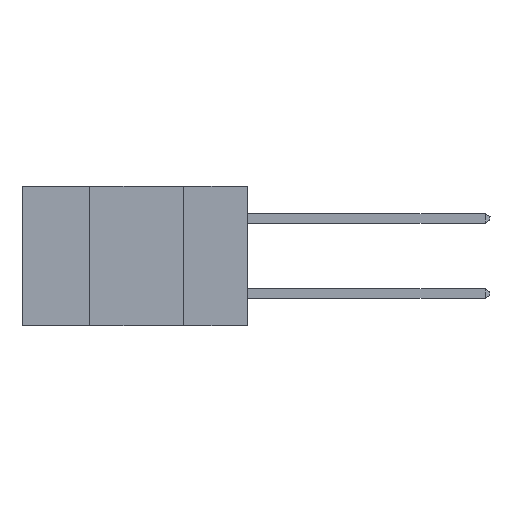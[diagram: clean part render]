
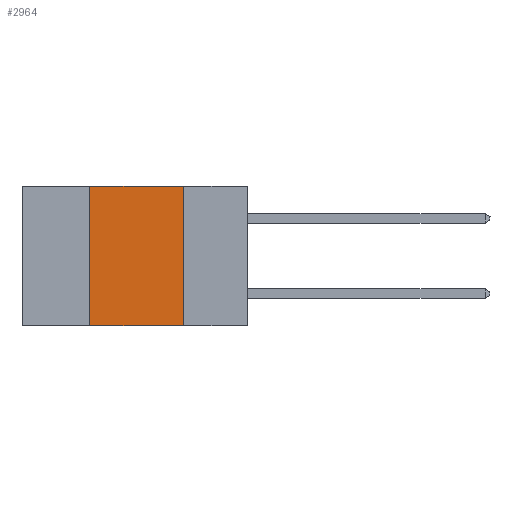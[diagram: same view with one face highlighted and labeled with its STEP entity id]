
A CAD part, left-side view. The second image highlights one B-rep face of the part: STEP entity #2964.
In plain terms, the highlighted planar face has unit normal (-1, 0, 0).
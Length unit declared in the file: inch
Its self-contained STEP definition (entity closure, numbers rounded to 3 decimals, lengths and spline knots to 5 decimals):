
#119 = DIRECTION ( 'NONE',  ( 0., -1., 0. ) ) ;
#792 = VECTOR ( 'NONE', #4960, 39.37008 ) ;
#814 = PLANE ( 'NONE',  #4036 ) ;
#1105 = ORIENTED_EDGE ( 'NONE', *, *, #10908, .F. ) ;
#1629 = EDGE_CURVE ( 'NONE', #7614, #4174, #7668, .T. ) ;
#1690 = DIRECTION ( 'NONE',  ( 0., -1., 0. ) ) ;
#1765 = DIRECTION ( 'NONE',  ( 1., 0., 0. ) ) ;
#1838 = CARTESIAN_POINT ( 'NONE',  ( 0., 0.42, 0. ) ) ;
#2436 = ORIENTED_EDGE ( 'NONE', *, *, #1629, .F. ) ;
#2517 = EDGE_CURVE ( 'NONE', #7547, #3492, #9523, .T. ) ;
#2719 = FACE_OUTER_BOUND ( 'NONE', #5638, .T. ) ;
#2964 = ADVANCED_FACE ( 'NONE', ( #2719 ), #814, .F. ) ;
#3097 = CARTESIAN_POINT ( 'NONE',  ( 0., 0.17, -0.37 ) ) ;
#3125 = CARTESIAN_POINT ( 'NONE',  ( 0., 0.42, -0.37 ) ) ;
#3251 = DIRECTION ( 'NONE',  ( 0., 0., 1. ) ) ;
#3470 = VECTOR ( 'NONE', #119, 39.37008 ) ;
#3492 = VERTEX_POINT ( 'NONE', #4029 ) ;
#3635 = EDGE_CURVE ( 'NONE', #7614, #3492, #7477, .T. ) ;
#4029 = CARTESIAN_POINT ( 'NONE',  ( 0., 0.17, -0.37 ) ) ;
#4036 = AXIS2_PLACEMENT_3D ( 'NONE', #8968, #1765, #5299 ) ;
#4174 = VERTEX_POINT ( 'NONE', #1838 ) ;
#4931 = ORIENTED_EDGE ( 'NONE', *, *, #3635, .T. ) ;
#4960 = DIRECTION ( 'NONE',  ( 0., 0., -1. ) ) ;
#5299 = DIRECTION ( 'NONE',  ( 0., 0., -1. ) ) ;
#5638 = EDGE_LOOP ( 'NONE', ( #11481, #1105, #2436, #4931 ) ) ;
#6113 = LINE ( 'NONE', #7183, #11177 ) ;
#7183 = CARTESIAN_POINT ( 'NONE',  ( 0., 0.6, 0. ) ) ;
#7477 = LINE ( 'NONE', #8176, #3470 ) ;
#7547 = VERTEX_POINT ( 'NONE', #9244 ) ;
#7614 = VERTEX_POINT ( 'NONE', #7764 ) ;
#7668 = LINE ( 'NONE', #3125, #11042 ) ;
#7764 = CARTESIAN_POINT ( 'NONE',  ( 0., 0.42, -0.37 ) ) ;
#8176 = CARTESIAN_POINT ( 'NONE',  ( 0., 0.6, -0.37 ) ) ;
#8968 = CARTESIAN_POINT ( 'NONE',  ( 0., 0.6, 0. ) ) ;
#9244 = CARTESIAN_POINT ( 'NONE',  ( 0., 0.17, 0. ) ) ;
#9523 = LINE ( 'NONE', #3097, #792 ) ;
#10908 = EDGE_CURVE ( 'NONE', #4174, #7547, #6113, .T. ) ;
#11042 = VECTOR ( 'NONE', #3251, 39.37008 ) ;
#11177 = VECTOR ( 'NONE', #1690, 39.37008 ) ;
#11481 = ORIENTED_EDGE ( 'NONE', *, *, #2517, .F. ) ;
